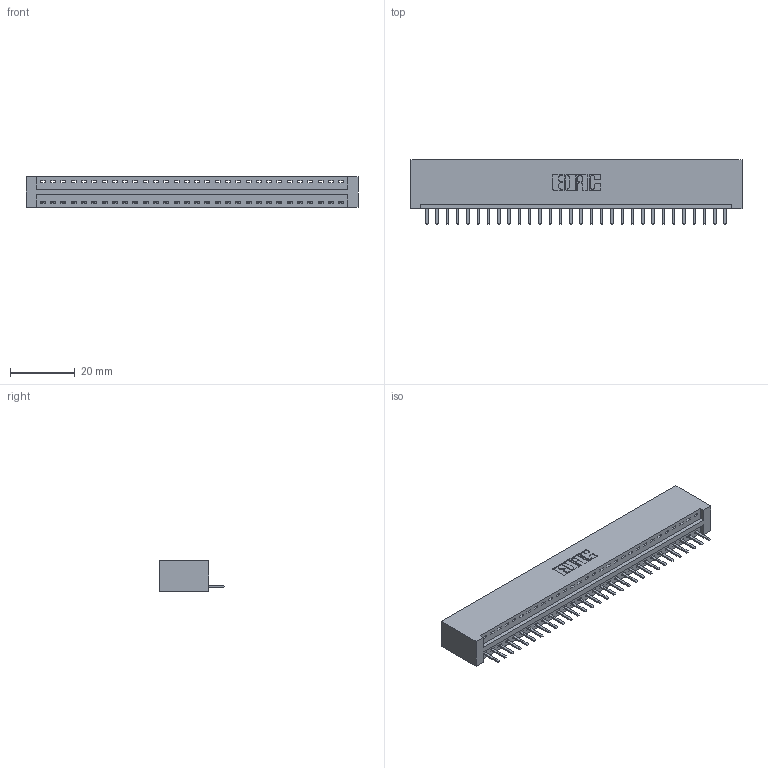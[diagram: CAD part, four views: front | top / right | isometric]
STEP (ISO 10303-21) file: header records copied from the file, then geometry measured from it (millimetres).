
FILE_DESCRIPTION (( 'STEP AP203' ), '1' );
FILE_NAME ('346-030-520-101.STEP', '2022-05-06T15:15:34', ( '' ), ( '' ), 'SwSTEP 2.0', 'SolidWorks 2020', '' );
FILE_SCHEMA (( 'CONFIG_CONTROL_DESIGN' ));
Length unit declared in the file: inch
Products named in the file (3): 346 Part_No Mounting Lugs; 346-030-520-101; 345-292-001_345-293-120
Assembly tree (31 placements, depth 2):
  346-030-520-101
    346 Part_No Mounting Lugs
    345-292-001_345-293-120  x30
Bounding box: 102.49 x 20.02 x 9.4 mm (x, y, z)
Volume: 10190.9 mm3; surface area: 12394.9 mm2
Topology: 31 solids, 31 shells, 1974 faces, 5825 edges, 3802 vertices
Faces by surface type: plane 1332, cylinder 642
Entity records: 20071 total; most frequent: CARTESIAN_POINT 3462, ORIENTED_EDGE 3414, DIRECTION 3051, EDGE_CURVE 1707, VECTOR 1459, LINE 1459, VERTEX_POINT 1134, AXIS2_PLACEMENT_3D 796
